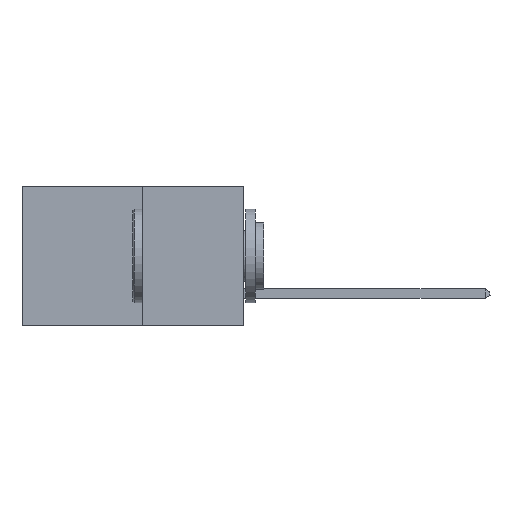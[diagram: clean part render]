
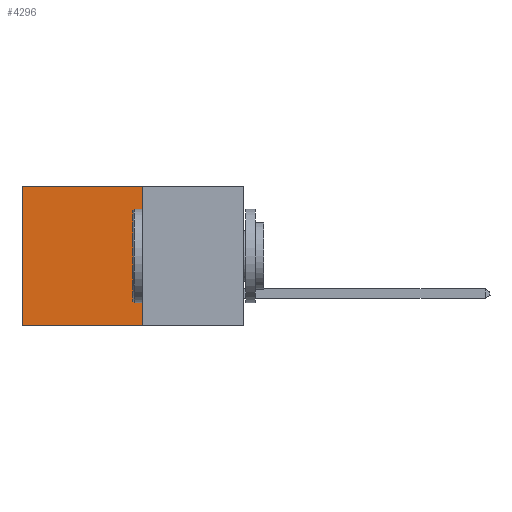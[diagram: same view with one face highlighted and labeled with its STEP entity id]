
A CAD part, left-side view. The second image highlights one B-rep face of the part: STEP entity #4296.
In plain terms, the highlighted planar face has unit normal (-1, 0, 0).
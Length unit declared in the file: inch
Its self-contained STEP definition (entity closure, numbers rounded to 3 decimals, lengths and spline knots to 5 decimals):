
#266 = EDGE_LOOP ( 'NONE', ( #13920, #11136, #7943, #8016 ) ) ;
#379 = EDGE_CURVE ( 'NONE', #2581, #10908, #1704, .T. ) ;
#555 = EDGE_CURVE ( 'NONE', #5820, #7954, #10369, .T. ) ;
#900 = EDGE_CURVE ( 'NONE', #7954, #10908, #9035, .T. ) ;
#1289 = VECTOR ( 'NONE', #2870, 39.37008 ) ;
#1383 = PLANE ( 'NONE',  #7915 ) ;
#1395 = EDGE_CURVE ( 'NONE', #5820, #2581, #13002, .T. ) ;
#1704 = LINE ( 'NONE', #12679, #7315 ) ;
#2581 = VERTEX_POINT ( 'NONE', #10127 ) ;
#2870 = DIRECTION ( 'NONE',  ( 0., 1., 0. ) ) ;
#4296 = ADVANCED_FACE ( 'NONE', ( #12571 ), #1383, .F. ) ;
#5820 = VERTEX_POINT ( 'NONE', #7197 ) ;
#6161 = DIRECTION ( 'NONE',  ( 0., 1., 0. ) ) ;
#6718 = CARTESIAN_POINT ( 'NONE',  ( 0.277, 0.27, -0.37 ) ) ;
#7197 = CARTESIAN_POINT ( 'NONE',  ( 0.277, 0.27, 0. ) ) ;
#7240 = DIRECTION ( 'NONE',  ( 0., 0., -1. ) ) ;
#7315 = VECTOR ( 'NONE', #6161, 39.37008 ) ;
#7567 = VECTOR ( 'NONE', #7240, 39.37008 ) ;
#7877 = DIRECTION ( 'NONE',  ( 0., 0., -1. ) ) ;
#7907 = DIRECTION ( 'NONE',  ( 1., 0., 0. ) ) ;
#7915 = AXIS2_PLACEMENT_3D ( 'NONE', #7946, #7907, #7877 ) ;
#7943 = ORIENTED_EDGE ( 'NONE', *, *, #1395, .F. ) ;
#7946 = CARTESIAN_POINT ( 'NONE',  ( 0.277, 0.27, -0.37 ) ) ;
#7954 = VERTEX_POINT ( 'NONE', #12224 ) ;
#8016 = ORIENTED_EDGE ( 'NONE', *, *, #555, .T. ) ;
#8240 = CARTESIAN_POINT ( 'NONE',  ( 0.277, 0.59, -0.37 ) ) ;
#8709 = VECTOR ( 'NONE', #9282, 39.37008 ) ;
#9035 = LINE ( 'NONE', #8240, #8709 ) ;
#9282 = DIRECTION ( 'NONE',  ( 0., 0., -1. ) ) ;
#10127 = CARTESIAN_POINT ( 'NONE',  ( 0.277, 0.27, -0.37 ) ) ;
#10369 = LINE ( 'NONE', #11407, #1289 ) ;
#10908 = VERTEX_POINT ( 'NONE', #11737 ) ;
#11136 = ORIENTED_EDGE ( 'NONE', *, *, #379, .F. ) ;
#11407 = CARTESIAN_POINT ( 'NONE',  ( 0.277, 0.27, 0. ) ) ;
#11737 = CARTESIAN_POINT ( 'NONE',  ( 0.277, 0.59, -0.37 ) ) ;
#12224 = CARTESIAN_POINT ( 'NONE',  ( 0.277, 0.59, 0. ) ) ;
#12571 = FACE_OUTER_BOUND ( 'NONE', #266, .T. ) ;
#12679 = CARTESIAN_POINT ( 'NONE',  ( 0.277, 0.27, -0.37 ) ) ;
#13002 = LINE ( 'NONE', #6718, #7567 ) ;
#13920 = ORIENTED_EDGE ( 'NONE', *, *, #900, .T. ) ;
